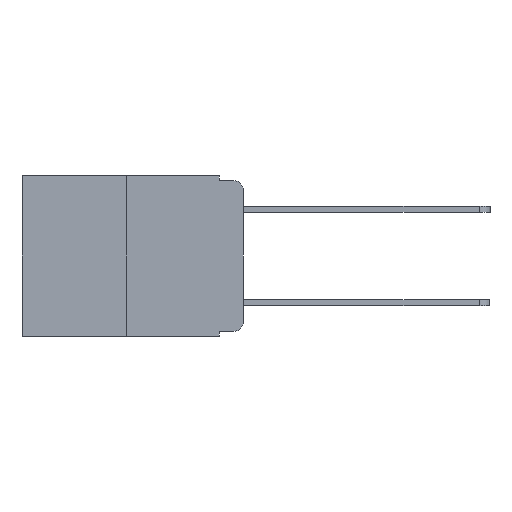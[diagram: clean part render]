
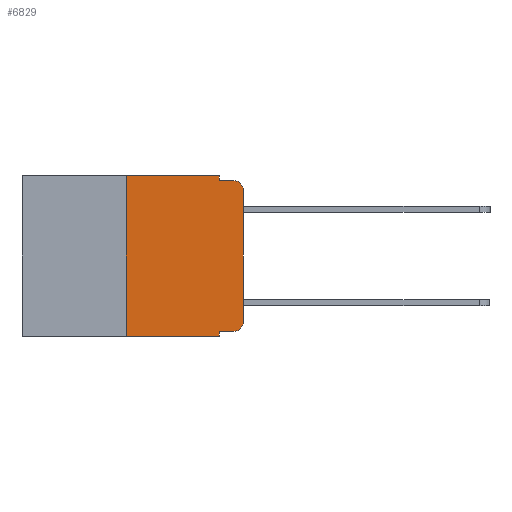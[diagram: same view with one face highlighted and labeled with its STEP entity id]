
A CAD part, left-side view. The second image highlights one B-rep face of the part: STEP entity #6829.
In plain terms, the highlighted planar face has unit normal (-1, 0, 0).
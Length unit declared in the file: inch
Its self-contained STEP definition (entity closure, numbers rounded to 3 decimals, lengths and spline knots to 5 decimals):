
#27 = DIRECTION ( 'NONE',  ( 0., -1., 0. ) ) ;
#64 = AXIS2_PLACEMENT_3D ( 'NONE', #9579, #5432, #5540 ) ;
#321 = CIRCLE ( 'NONE', #64, 0.02 ) ;
#421 = VERTEX_POINT ( 'NONE', #10898 ) ;
#787 = ORIENTED_EDGE ( 'NONE', *, *, #8183, .T. ) ;
#965 = DIRECTION ( 'NONE',  ( -1., 0., 0. ) ) ;
#972 = LINE ( 'NONE', #11398, #5502 ) ;
#991 = VERTEX_POINT ( 'NONE', #9099 ) ;
#993 = ORIENTED_EDGE ( 'NONE', *, *, #6504, .F. ) ;
#1238 = CIRCLE ( 'NONE', #9387, 0.02 ) ;
#1369 = ORIENTED_EDGE ( 'NONE', *, *, #7655, .F. ) ;
#2498 = CARTESIAN_POINT ( 'NONE',  ( 0., 0., 0. ) ) ;
#2877 = ORIENTED_EDGE ( 'NONE', *, *, #8720, .T. ) ;
#2912 = CARTESIAN_POINT ( 'NONE',  ( 0., 0.473, 0. ) ) ;
#3133 = VERTEX_POINT ( 'NONE', #6659 ) ;
#3374 = DIRECTION ( 'NONE',  ( 0., 0., 1. ) ) ;
#3431 = DIRECTION ( 'NONE',  ( 0., -1., 0. ) ) ;
#3472 = VECTOR ( 'NONE', #9077, 39.37008 ) ;
#3553 = ORIENTED_EDGE ( 'NONE', *, *, #4631, .T. ) ;
#3596 = CARTESIAN_POINT ( 'NONE',  ( 0., 0.25, -0.343 ) ) ;
#3883 = DIRECTION ( 'NONE',  ( 0., -1., 0. ) ) ;
#4012 = FACE_OUTER_BOUND ( 'NONE', #6142, .T. ) ;
#4502 = ORIENTED_EDGE ( 'NONE', *, *, #7076, .F. ) ;
#4549 = CARTESIAN_POINT ( 'NONE',  ( 0., 0.051, -0.01 ) ) ;
#4631 = EDGE_CURVE ( 'NONE', #3133, #9856, #321, .T. ) ;
#4645 = CARTESIAN_POINT ( 'NONE',  ( 0., 0.02, -0.01 ) ) ;
#4688 = ORIENTED_EDGE ( 'NONE', *, *, #8471, .F. ) ;
#4825 = CARTESIAN_POINT ( 'NONE',  ( 0., 0., -0.313 ) ) ;
#4880 = VERTEX_POINT ( 'NONE', #6105 ) ;
#5136 = CARTESIAN_POINT ( 'NONE',  ( 0., 0.051, -0.01 ) ) ;
#5170 = VECTOR ( 'NONE', #3374, 39.37008 ) ;
#5265 = EDGE_CURVE ( 'NONE', #4880, #3133, #6526, .T. ) ;
#5432 = DIRECTION ( 'NONE',  ( -1., 0., 0. ) ) ;
#5502 = VECTOR ( 'NONE', #3431, 39.37008 ) ;
#5540 = DIRECTION ( 'NONE',  ( 0., 0., -1. ) ) ;
#5751 = LINE ( 'NONE', #7985, #10508 ) ;
#5870 = EDGE_CURVE ( 'NONE', #4880, #7016, #10402, .T. ) ;
#5905 = ORIENTED_EDGE ( 'NONE', *, *, #5265, .T. ) ;
#6105 = CARTESIAN_POINT ( 'NONE',  ( 0., 0.051, -0.333 ) ) ;
#6142 = EDGE_LOOP ( 'NONE', ( #2877, #787, #1369, #4502, #4688, #993, #11683, #7845, #5905, #3553 ) ) ;
#6149 = EDGE_CURVE ( 'NONE', #6180, #7016, #972, .T. ) ;
#6180 = VERTEX_POINT ( 'NONE', #3596 ) ;
#6275 = CARTESIAN_POINT ( 'NONE',  ( 0., 0.051, -0.333 ) ) ;
#6403 = DIRECTION ( 'NONE',  ( 0., -1., 0. ) ) ;
#6504 = EDGE_CURVE ( 'NONE', #6180, #7159, #7717, .T. ) ;
#6526 = LINE ( 'NONE', #6275, #8469 ) ;
#6659 = CARTESIAN_POINT ( 'NONE',  ( 0., 0.02, -0.333 ) ) ;
#6829 = ADVANCED_FACE ( 'NONE', ( #4012 ), #9384, .F. ) ;
#7016 = VERTEX_POINT ( 'NONE', #11202 ) ;
#7076 = EDGE_CURVE ( 'NONE', #991, #10484, #5751, .T. ) ;
#7146 = LINE ( 'NONE', #2912, #11261 ) ;
#7159 = VERTEX_POINT ( 'NONE', #7642 ) ;
#7175 = VECTOR ( 'NONE', #3883, 39.37008 ) ;
#7538 = LINE ( 'NONE', #2498, #5170 ) ;
#7642 = CARTESIAN_POINT ( 'NONE',  ( 0., 0.25, 0. ) ) ;
#7655 = EDGE_CURVE ( 'NONE', #10484, #10509, #9344, .T. ) ;
#7717 = LINE ( 'NONE', #10369, #9351 ) ;
#7845 = ORIENTED_EDGE ( 'NONE', *, *, #5870, .F. ) ;
#7946 = DIRECTION ( 'NONE',  ( 0., 0., -1. ) ) ;
#7985 = CARTESIAN_POINT ( 'NONE',  ( 0., 0.051, 0. ) ) ;
#8007 = DIRECTION ( 'NONE',  ( 0., 0., -1. ) ) ;
#8183 = EDGE_CURVE ( 'NONE', #421, #10509, #1238, .T. ) ;
#8469 = VECTOR ( 'NONE', #6403, 39.37008 ) ;
#8471 = EDGE_CURVE ( 'NONE', #7159, #991, #7146, .T. ) ;
#8541 = AXIS2_PLACEMENT_3D ( 'NONE', #10696, #10565, #10538 ) ;
#8686 = CARTESIAN_POINT ( 'NONE',  ( 0., 0.051, 0. ) ) ;
#8720 = EDGE_CURVE ( 'NONE', #9856, #421, #7538, .T. ) ;
#9077 = DIRECTION ( 'NONE',  ( 0., 0., -1. ) ) ;
#9099 = CARTESIAN_POINT ( 'NONE',  ( 0., 0.051, 0. ) ) ;
#9344 = LINE ( 'NONE', #5136, #7175 ) ;
#9346 = CARTESIAN_POINT ( 'NONE',  ( 0., 0.02, -0.03 ) ) ;
#9351 = VECTOR ( 'NONE', #11580, 39.37008 ) ;
#9384 = PLANE ( 'NONE',  #8541 ) ;
#9387 = AXIS2_PLACEMENT_3D ( 'NONE', #9346, #965, #8007 ) ;
#9579 = CARTESIAN_POINT ( 'NONE',  ( 0., 0.02, -0.313 ) ) ;
#9856 = VERTEX_POINT ( 'NONE', #4825 ) ;
#10369 = CARTESIAN_POINT ( 'NONE',  ( 0., 0.25, 0. ) ) ;
#10402 = LINE ( 'NONE', #8686, #3472 ) ;
#10484 = VERTEX_POINT ( 'NONE', #4549 ) ;
#10508 = VECTOR ( 'NONE', #7946, 39.37008 ) ;
#10509 = VERTEX_POINT ( 'NONE', #4645 ) ;
#10538 = DIRECTION ( 'NONE',  ( 0., 0., -1. ) ) ;
#10565 = DIRECTION ( 'NONE',  ( 1., 0., 0. ) ) ;
#10696 = CARTESIAN_POINT ( 'NONE',  ( 0., 0.473, 0. ) ) ;
#10898 = CARTESIAN_POINT ( 'NONE',  ( 0., 0., -0.03 ) ) ;
#11202 = CARTESIAN_POINT ( 'NONE',  ( 0., 0.051, -0.343 ) ) ;
#11261 = VECTOR ( 'NONE', #27, 39.37008 ) ;
#11398 = CARTESIAN_POINT ( 'NONE',  ( 0., 0.473, -0.343 ) ) ;
#11580 = DIRECTION ( 'NONE',  ( 0., 0., 1. ) ) ;
#11683 = ORIENTED_EDGE ( 'NONE', *, *, #6149, .T. ) ;
